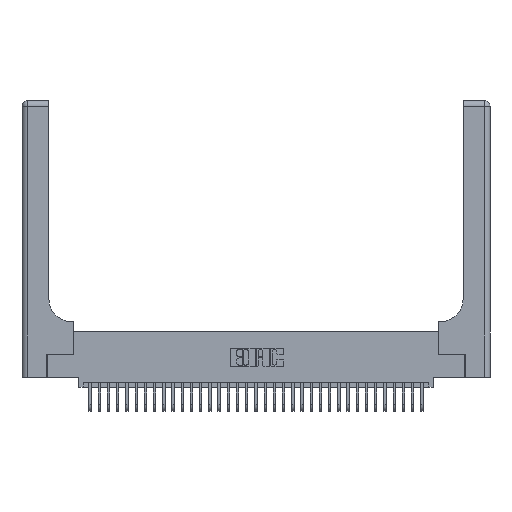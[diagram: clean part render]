
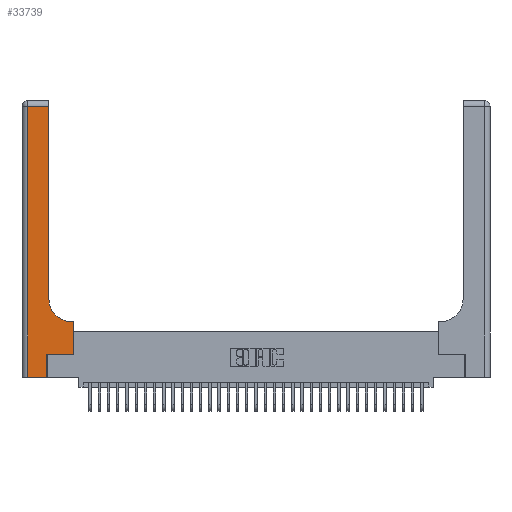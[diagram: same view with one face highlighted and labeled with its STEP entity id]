
A CAD part, top view. The second image highlights one B-rep face of the part: STEP entity #33739.
In plain terms, the highlighted planar face has unit normal (0, 0, 1).
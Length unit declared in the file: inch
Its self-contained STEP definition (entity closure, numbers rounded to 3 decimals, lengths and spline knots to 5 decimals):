
#609 = CARTESIAN_POINT ( 'NONE',  ( 0.5415, 0.6, 0.37 ) ) ;
#614 = VERTEX_POINT ( 'NONE', #33328 ) ;
#977 = ORIENTED_EDGE ( 'NONE', *, *, #9536, .T. ) ;
#1807 = ORIENTED_EDGE ( 'NONE', *, *, #21768, .T. ) ;
#2187 = CARTESIAN_POINT ( 'NONE',  ( 0., 0., 0.37 ) ) ;
#2489 = VERTEX_POINT ( 'NONE', #25473 ) ;
#2686 = EDGE_CURVE ( 'NONE', #12794, #13502, #22277, .T. ) ;
#2872 = CARTESIAN_POINT ( 'NONE',  ( 0.06, 2.94, 0.37 ) ) ;
#2898 = ORIENTED_EDGE ( 'NONE', *, *, #14448, .T. ) ;
#2995 = ORIENTED_EDGE ( 'NONE', *, *, #15027, .T. ) ;
#3245 = CARTESIAN_POINT ( 'NONE',  ( 0.5415, 0.85, 0.37 ) ) ;
#3539 = CARTESIAN_POINT ( 'NONE',  ( 0., 2.94, 0.37 ) ) ;
#3854 = CARTESIAN_POINT ( 'NONE',  ( 0.5585, 0.25, 0.37 ) ) ;
#4205 = AXIS2_PLACEMENT_3D ( 'NONE', #3245, #21669, #5933 ) ;
#4401 = VERTEX_POINT ( 'NONE', #609 ) ;
#4724 = LINE ( 'NONE', #28777, #11003 ) ;
#4831 = ORIENTED_EDGE ( 'NONE', *, *, #22002, .T. ) ;
#5933 = DIRECTION ( 'NONE',  ( 1., 0., 0. ) ) ;
#5951 = VECTOR ( 'NONE', #11069, 39.37008 ) ;
#7585 = CARTESIAN_POINT ( 'NONE',  ( 0.2915, 0.85, 0.37 ) ) ;
#7946 = CARTESIAN_POINT ( 'NONE',  ( 0.2915, 3., 0.37 ) ) ;
#8422 = VECTOR ( 'NONE', #21104, 39.37008 ) ;
#9536 = EDGE_CURVE ( 'NONE', #13502, #33226, #15762, .T. ) ;
#9798 = ORIENTED_EDGE ( 'NONE', *, *, #18937, .T. ) ;
#10348 = CARTESIAN_POINT ( 'NONE',  ( 0., 3., 0.37 ) ) ;
#10385 = CARTESIAN_POINT ( 'NONE',  ( 0.06, 3., 0.37 ) ) ;
#11003 = VECTOR ( 'NONE', #13303, 39.37008 ) ;
#11069 = DIRECTION ( 'NONE',  ( 1., 0., 0. ) ) ;
#11450 = ORIENTED_EDGE ( 'NONE', *, *, #23492, .T. ) ;
#11461 = LINE ( 'NONE', #10385, #32138 ) ;
#12607 = CARTESIAN_POINT ( 'NONE',  ( 0.269, 0., 0.37 ) ) ;
#12794 = VERTEX_POINT ( 'NONE', #7585 ) ;
#12810 = ORIENTED_EDGE ( 'NONE', *, *, #2686, .T. ) ;
#13007 = DIRECTION ( 'NONE',  ( -1., 0., 0. ) ) ;
#13303 = DIRECTION ( 'NONE',  ( 0., 1., 0. ) ) ;
#13502 = VERTEX_POINT ( 'NONE', #21066 ) ;
#13642 = CARTESIAN_POINT ( 'NONE',  ( 0.269, 0.25, 0.37 ) ) ;
#13897 = LINE ( 'NONE', #13642, #5951 ) ;
#14156 = VECTOR ( 'NONE', #15456, 39.37008 ) ;
#14407 = CARTESIAN_POINT ( 'NONE',  ( 0.269, 0.25, 0.37 ) ) ;
#14448 = EDGE_CURVE ( 'NONE', #21704, #28939, #16424, .T. ) ;
#14944 = VECTOR ( 'NONE', #19330, 39.37008 ) ;
#15027 = EDGE_CURVE ( 'NONE', #33226, #614, #11461, .T. ) ;
#15456 = DIRECTION ( 'NONE',  ( 1., 0., 0. ) ) ;
#15607 = VECTOR ( 'NONE', #22782, 39.37008 ) ;
#15762 = LINE ( 'NONE', #3539, #14944 ) ;
#16424 = LINE ( 'NONE', #22661, #15607 ) ;
#17317 = DIRECTION ( 'NONE',  ( -1., 0., 0. ) ) ;
#18937 = EDGE_CURVE ( 'NONE', #2489, #4401, #32087, .T. ) ;
#19330 = DIRECTION ( 'NONE',  ( -1., 0., 0. ) ) ;
#21066 = CARTESIAN_POINT ( 'NONE',  ( 0.2915, 2.94, 0.37 ) ) ;
#21104 = DIRECTION ( 'NONE',  ( 0., 1., 0. ) ) ;
#21408 = CIRCLE ( 'NONE', #4205, 0.25 ) ;
#21553 = VERTEX_POINT ( 'NONE', #3854 ) ;
#21669 = DIRECTION ( 'NONE',  ( 0., 0., -1. ) ) ;
#21704 = VERTEX_POINT ( 'NONE', #12607 ) ;
#21768 = EDGE_CURVE ( 'NONE', #614, #21704, #27889, .T. ) ;
#22002 = EDGE_CURVE ( 'NONE', #4401, #12794, #21408, .T. ) ;
#22277 = LINE ( 'NONE', #7946, #8422 ) ;
#22297 = ORIENTED_EDGE ( 'NONE', *, *, #33250, .T. ) ;
#22418 = CARTESIAN_POINT ( 'NONE',  ( 0.2915, 0.6, 0.37 ) ) ;
#22661 = CARTESIAN_POINT ( 'NONE',  ( 0.269, 0., 0.37 ) ) ;
#22782 = DIRECTION ( 'NONE',  ( 0., 1., 0. ) ) ;
#23492 = EDGE_CURVE ( 'NONE', #21553, #2489, #4724, .T. ) ;
#25184 = VECTOR ( 'NONE', #17317, 39.37008 ) ;
#25473 = CARTESIAN_POINT ( 'NONE',  ( 0.5585, 0.6, 0.37 ) ) ;
#25963 = FACE_OUTER_BOUND ( 'NONE', #28760, .T. ) ;
#27889 = LINE ( 'NONE', #2187, #14156 ) ;
#28408 = AXIS2_PLACEMENT_3D ( 'NONE', #10348, #28512, #13007 ) ;
#28512 = DIRECTION ( 'NONE',  ( 0., 0., -1. ) ) ;
#28548 = DIRECTION ( 'NONE',  ( 0., -1., 0. ) ) ;
#28760 = EDGE_LOOP ( 'NONE', ( #12810, #977, #2995, #1807, #2898, #22297, #11450, #9798, #4831 ) ) ;
#28777 = CARTESIAN_POINT ( 'NONE',  ( 0.5585, 0.25, 0.37 ) ) ;
#28939 = VERTEX_POINT ( 'NONE', #14407 ) ;
#30999 = PLANE ( 'NONE',  #28408 ) ;
#32087 = LINE ( 'NONE', #22418, #25184 ) ;
#32138 = VECTOR ( 'NONE', #28548, 39.37008 ) ;
#33226 = VERTEX_POINT ( 'NONE', #2872 ) ;
#33250 = EDGE_CURVE ( 'NONE', #28939, #21553, #13897, .T. ) ;
#33328 = CARTESIAN_POINT ( 'NONE',  ( 0.06, 0., 0.37 ) ) ;
#33739 = ADVANCED_FACE ( 'NONE', ( #25963 ), #30999, .F. ) ;
